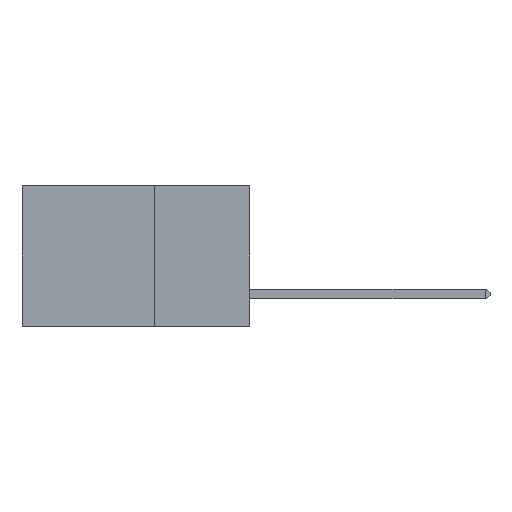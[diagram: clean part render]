
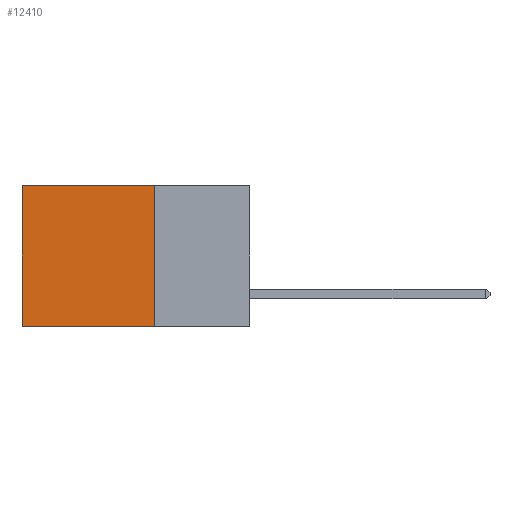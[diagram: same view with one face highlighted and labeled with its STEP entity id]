
A CAD part, left-side view. The second image highlights one B-rep face of the part: STEP entity #12410.
In plain terms, the highlighted planar face has unit normal (-1, 0, 0).
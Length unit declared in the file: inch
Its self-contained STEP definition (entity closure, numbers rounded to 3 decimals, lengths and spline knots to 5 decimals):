
#713 = LINE ( 'NONE', #1313, #6869 ) ;
#996 = EDGE_CURVE ( 'NONE', #7382, #7014, #1389, .T. ) ;
#1120 = DIRECTION ( 'NONE',  ( 0., 1., 0. ) ) ;
#1140 = EDGE_CURVE ( 'NONE', #7014, #12697, #4850, .T. ) ;
#1157 = CARTESIAN_POINT ( 'NONE',  ( 0.2875, 0.25, 0. ) ) ;
#1194 = VECTOR ( 'NONE', #15321, 39.37008 ) ;
#1313 = CARTESIAN_POINT ( 'NONE',  ( 0.2875, 0.6, 0. ) ) ;
#1389 = LINE ( 'NONE', #15247, #6770 ) ;
#1798 = CARTESIAN_POINT ( 'NONE',  ( 0.2875, 0.6, -0.37 ) ) ;
#2409 = EDGE_CURVE ( 'NONE', #7382, #7188, #6333, .T. ) ;
#2686 = VECTOR ( 'NONE', #1120, 39.37008 ) ;
#3439 = FACE_OUTER_BOUND ( 'NONE', #9951, .T. ) ;
#3702 = DIRECTION ( 'NONE',  ( 1., 0., 0. ) ) ;
#4850 = LINE ( 'NONE', #11608, #1194 ) ;
#4884 = CARTESIAN_POINT ( 'NONE',  ( 0.2875, 0.25, 0. ) ) ;
#6333 = LINE ( 'NONE', #1157, #2686 ) ;
#6397 = ORIENTED_EDGE ( 'NONE', *, *, #996, .F. ) ;
#6770 = VECTOR ( 'NONE', #13894, 39.37008 ) ;
#6869 = VECTOR ( 'NONE', #7482, 39.37008 ) ;
#7014 = VERTEX_POINT ( 'NONE', #8611 ) ;
#7188 = VERTEX_POINT ( 'NONE', #10027 ) ;
#7382 = VERTEX_POINT ( 'NONE', #15073 ) ;
#7482 = DIRECTION ( 'NONE',  ( 0., 0., -1. ) ) ;
#8534 = PLANE ( 'NONE',  #12423 ) ;
#8611 = CARTESIAN_POINT ( 'NONE',  ( 0.2875, 0.25, -0.37 ) ) ;
#9789 = ORIENTED_EDGE ( 'NONE', *, *, #2409, .T. ) ;
#9951 = EDGE_LOOP ( 'NONE', ( #13021, #14567, #6397, #9789 ) ) ;
#10027 = CARTESIAN_POINT ( 'NONE',  ( 0.2875, 0.6, 0. ) ) ;
#11608 = CARTESIAN_POINT ( 'NONE',  ( 0.2875, 0.25, -0.37 ) ) ;
#12019 = DIRECTION ( 'NONE',  ( 0., 0., -1. ) ) ;
#12410 = ADVANCED_FACE ( 'NONE', ( #3439 ), #8534, .F. ) ;
#12423 = AXIS2_PLACEMENT_3D ( 'NONE', #4884, #3702, #12019 ) ;
#12697 = VERTEX_POINT ( 'NONE', #1798 ) ;
#12971 = EDGE_CURVE ( 'NONE', #7188, #12697, #713, .T. ) ;
#13021 = ORIENTED_EDGE ( 'NONE', *, *, #12971, .T. ) ;
#13894 = DIRECTION ( 'NONE',  ( 0., 0., -1. ) ) ;
#14567 = ORIENTED_EDGE ( 'NONE', *, *, #1140, .F. ) ;
#15073 = CARTESIAN_POINT ( 'NONE',  ( 0.2875, 0.25, 0. ) ) ;
#15247 = CARTESIAN_POINT ( 'NONE',  ( 0.2875, 0.25, 0. ) ) ;
#15321 = DIRECTION ( 'NONE',  ( 0., 1., 0. ) ) ;
